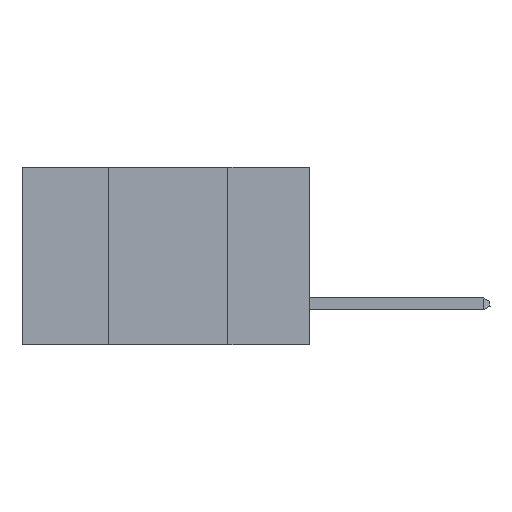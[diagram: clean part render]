
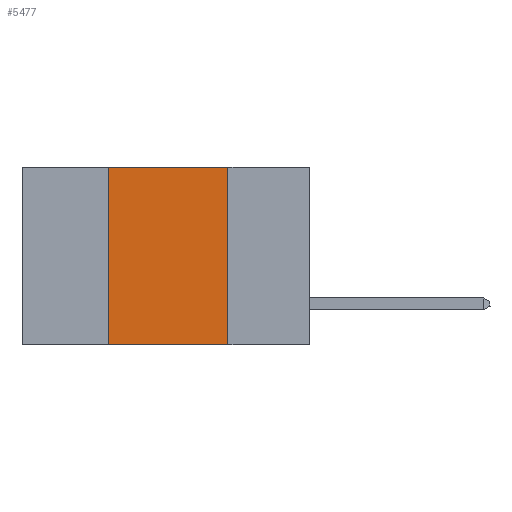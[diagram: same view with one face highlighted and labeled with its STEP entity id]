
A CAD part, left-side view. The second image highlights one B-rep face of the part: STEP entity #5477.
In plain terms, the highlighted planar face has unit normal (-1, 0, 0).
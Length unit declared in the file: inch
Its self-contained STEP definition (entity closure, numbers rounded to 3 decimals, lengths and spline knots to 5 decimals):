
#66 = VECTOR ( 'NONE', #1002, 39.37008 ) ;
#256 = DIRECTION ( 'NONE',  ( 0., -1., 0. ) ) ;
#357 = CARTESIAN_POINT ( 'NONE',  ( 0., 0.17, -0.37 ) ) ;
#481 = EDGE_CURVE ( 'NONE', #6000, #6556, #5647, .T. ) ;
#553 = DIRECTION ( 'NONE',  ( 0., 0., 1. ) ) ;
#717 = EDGE_CURVE ( 'NONE', #11025, #5843, #8835, .T. ) ;
#869 = DIRECTION ( 'NONE',  ( 0., 0., -1. ) ) ;
#1002 = DIRECTION ( 'NONE',  ( 0., 0., -1. ) ) ;
#1145 = LINE ( 'NONE', #7142, #6438 ) ;
#1357 = CARTESIAN_POINT ( 'NONE',  ( 0., 0.42, -0.37 ) ) ;
#1517 = AXIS2_PLACEMENT_3D ( 'NONE', #1889, #4843, #869 ) ;
#1606 = EDGE_LOOP ( 'NONE', ( #1669, #7430, #7136, #3231 ) ) ;
#1669 = ORIENTED_EDGE ( 'NONE', *, *, #481, .F. ) ;
#1889 = CARTESIAN_POINT ( 'NONE',  ( 0., 0.6, 0. ) ) ;
#2992 = EDGE_CURVE ( 'NONE', #11025, #6556, #4428, .T. ) ;
#3231 = ORIENTED_EDGE ( 'NONE', *, *, #2992, .T. ) ;
#4294 = DIRECTION ( 'NONE',  ( 0., -1., 0. ) ) ;
#4428 = LINE ( 'NONE', #11967, #4557 ) ;
#4557 = VECTOR ( 'NONE', #256, 39.37008 ) ;
#4843 = DIRECTION ( 'NONE',  ( 1., 0., 0. ) ) ;
#5067 = CARTESIAN_POINT ( 'NONE',  ( 0., 0.17, 0. ) ) ;
#5477 = ADVANCED_FACE ( 'NONE', ( #9327 ), #8693, .F. ) ;
#5489 = CARTESIAN_POINT ( 'NONE',  ( 0., 0.42, 0. ) ) ;
#5647 = LINE ( 'NONE', #5067, #66 ) ;
#5843 = VERTEX_POINT ( 'NONE', #6269 ) ;
#6000 = VERTEX_POINT ( 'NONE', #9056 ) ;
#6269 = CARTESIAN_POINT ( 'NONE',  ( 0., 0.42, 0. ) ) ;
#6438 = VECTOR ( 'NONE', #4294, 39.37008 ) ;
#6556 = VERTEX_POINT ( 'NONE', #357 ) ;
#7136 = ORIENTED_EDGE ( 'NONE', *, *, #717, .F. ) ;
#7142 = CARTESIAN_POINT ( 'NONE',  ( 0., 0.6, 0. ) ) ;
#7430 = ORIENTED_EDGE ( 'NONE', *, *, #10326, .F. ) ;
#8693 = PLANE ( 'NONE',  #1517 ) ;
#8835 = LINE ( 'NONE', #5489, #9450 ) ;
#9056 = CARTESIAN_POINT ( 'NONE',  ( 0., 0.17, 0. ) ) ;
#9327 = FACE_OUTER_BOUND ( 'NONE', #1606, .T. ) ;
#9450 = VECTOR ( 'NONE', #553, 39.37008 ) ;
#10326 = EDGE_CURVE ( 'NONE', #5843, #6000, #1145, .T. ) ;
#11025 = VERTEX_POINT ( 'NONE', #1357 ) ;
#11967 = CARTESIAN_POINT ( 'NONE',  ( 0., 0.6, -0.37 ) ) ;
